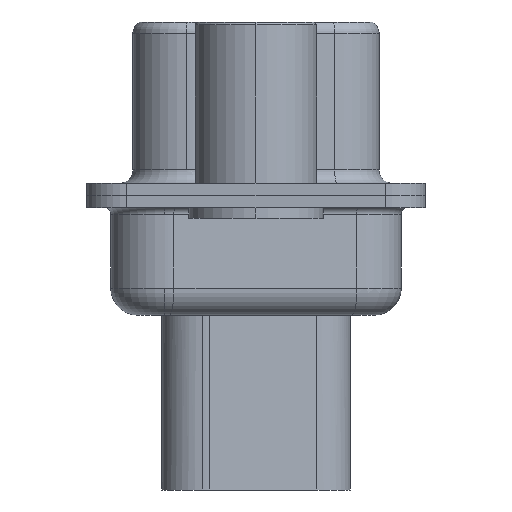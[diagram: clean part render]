
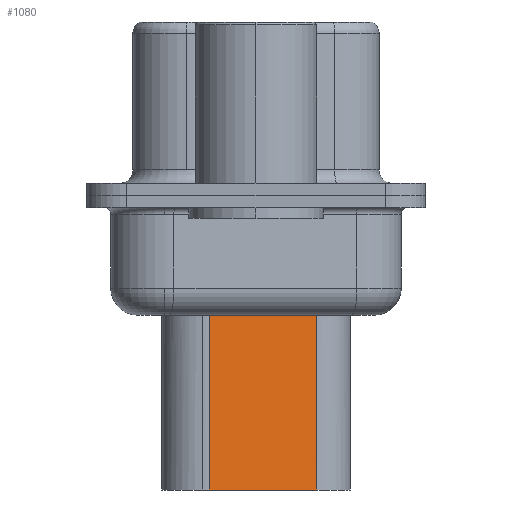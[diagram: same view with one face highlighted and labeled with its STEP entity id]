
A CAD part, left-side view. The second image highlights one B-rep face of the part: STEP entity #1080.
In plain terms, the highlighted planar face has unit normal (-0.985, -0.174, 0).
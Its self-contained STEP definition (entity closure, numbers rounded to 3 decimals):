
#87 = PLANE ( 'NONE',  #10787 ) ;
#580 = ORIENTED_EDGE ( 'NONE', *, *, #4774, .T. ) ;
#873 = EDGE_LOOP ( 'NONE', ( #1032, #580, #4032, #3257 ) ) ;
#897 = LINE ( 'NONE', #4976, #10440 ) ;
#1032 = ORIENTED_EDGE ( 'NONE', *, *, #2327, .F. ) ;
#1080 = ADVANCED_FACE ( 'NONE', ( #1892 ), #87, .T. ) ;
#1892 = FACE_OUTER_BOUND ( 'NONE', #873, .T. ) ;
#2327 = EDGE_CURVE ( 'NONE', #4733, #9785, #11088, .T. ) ;
#2805 = VERTEX_POINT ( 'NONE', #8305 ) ;
#2995 = CARTESIAN_POINT ( 'NONE',  ( 4.353, 2.709, -3.975 ) ) ;
#3257 = ORIENTED_EDGE ( 'NONE', *, *, #4772, .F. ) ;
#3935 = CARTESIAN_POINT ( 'NONE',  ( 4.524, 1.74, -3.1 ) ) ;
#4032 = ORIENTED_EDGE ( 'NONE', *, *, #7388, .T. ) ;
#4166 = VECTOR ( 'NONE', #5184, 1000. ) ;
#4192 = LINE ( 'NONE', #3935, #4166 ) ;
#4733 = VERTEX_POINT ( 'NONE', #8293 ) ;
#4772 = EDGE_CURVE ( 'NONE', #9785, #2805, #897, .T. ) ;
#4774 = EDGE_CURVE ( 'NONE', #4733, #5628, #12830, .T. ) ;
#4976 = CARTESIAN_POINT ( 'NONE',  ( 4.524, 1.74, -10.95 ) ) ;
#5184 = DIRECTION ( 'NONE',  ( 0., 0., -1. ) ) ;
#5222 = CARTESIAN_POINT ( 'NONE',  ( 4.524, 1.74, -3.975 ) ) ;
#5299 = CARTESIAN_POINT ( 'NONE',  ( 5.229, -2.26, -10.95 ) ) ;
#5628 = VERTEX_POINT ( 'NONE', #5222 ) ;
#6117 = DIRECTION ( 'NONE',  ( 0., 0., -1. ) ) ;
#6180 = VECTOR ( 'NONE', #6117, 1000. ) ;
#7388 = EDGE_CURVE ( 'NONE', #5628, #2805, #4192, .T. ) ;
#8110 = DIRECTION ( 'NONE',  ( 0.174, -0.985, 0. ) ) ;
#8293 = CARTESIAN_POINT ( 'NONE',  ( 5.229, -2.26, -3.975 ) ) ;
#8305 = CARTESIAN_POINT ( 'NONE',  ( 4.524, 1.74, -10.95 ) ) ;
#9027 = DIRECTION ( 'NONE',  ( -0.174, 0.985, 0. ) ) ;
#9082 = CARTESIAN_POINT ( 'NONE',  ( 4.524, 1.74, -3.1 ) ) ;
#9613 = VECTOR ( 'NONE', #11053, 1000. ) ;
#9785 = VERTEX_POINT ( 'NONE', #5299 ) ;
#10128 = DIRECTION ( 'NONE',  ( -0.985, -0.174, 0. ) ) ;
#10440 = VECTOR ( 'NONE', #9027, 1000. ) ;
#10787 = AXIS2_PLACEMENT_3D ( 'NONE', #9082, #10128, #8110 ) ;
#11053 = DIRECTION ( 'NONE',  ( -0.174, 0.985, 0. ) ) ;
#11088 = LINE ( 'NONE', #12074, #6180 ) ;
#12074 = CARTESIAN_POINT ( 'NONE',  ( 5.229, -2.26, -3.1 ) ) ;
#12830 = LINE ( 'NONE', #2995, #9613 ) ;
